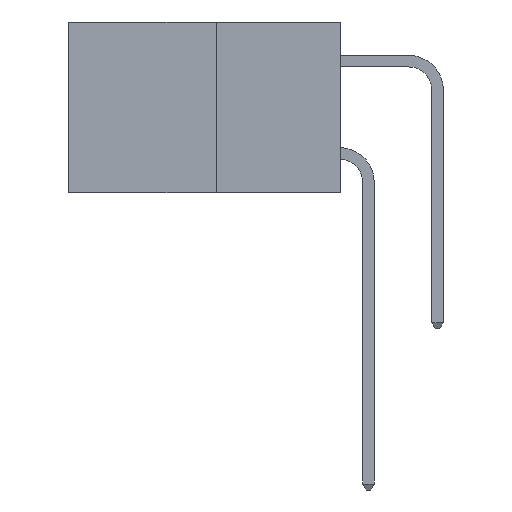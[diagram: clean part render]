
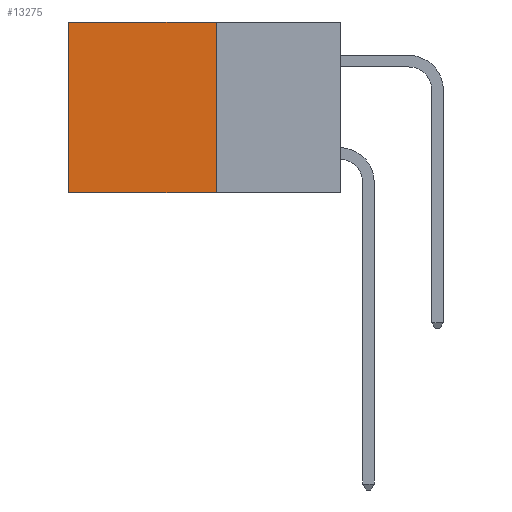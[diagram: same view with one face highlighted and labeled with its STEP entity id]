
A CAD part, left-side view. The second image highlights one B-rep face of the part: STEP entity #13275.
In plain terms, the highlighted planar face has unit normal (-1, 0, 0).
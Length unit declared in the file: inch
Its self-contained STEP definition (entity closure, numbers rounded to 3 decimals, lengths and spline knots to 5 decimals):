
#1402 = DIRECTION ( 'NONE',  ( 0., 0., -1. ) ) ;
#1432 = ORIENTED_EDGE ( 'NONE', *, *, #3267, .T. ) ;
#1830 = VERTEX_POINT ( 'NONE', #9430 ) ;
#2218 = CARTESIAN_POINT ( 'NONE',  ( 0.277, 0.59, -0.37 ) ) ;
#2800 = VERTEX_POINT ( 'NONE', #19745 ) ;
#2997 = VECTOR ( 'NONE', #15778, 39.37008 ) ;
#3267 = EDGE_CURVE ( 'NONE', #7674, #1830, #17263, .T. ) ;
#3533 = PLANE ( 'NONE',  #20308 ) ;
#3918 = FACE_OUTER_BOUND ( 'NONE', #11675, .T. ) ;
#4241 = VERTEX_POINT ( 'NONE', #22824 ) ;
#5569 = CARTESIAN_POINT ( 'NONE',  ( 0.277, 0.27, -0.37 ) ) ;
#5927 = CARTESIAN_POINT ( 'NONE',  ( 0.277, 0.27, 0. ) ) ;
#6633 = DIRECTION ( 'NONE',  ( 0., 1., 0. ) ) ;
#7389 = EDGE_CURVE ( 'NONE', #1830, #4241, #8307, .T. ) ;
#7457 = ORIENTED_EDGE ( 'NONE', *, *, #21465, .F. ) ;
#7630 = DIRECTION ( 'NONE',  ( 1., 0., 0. ) ) ;
#7674 = VERTEX_POINT ( 'NONE', #5927 ) ;
#8307 = LINE ( 'NONE', #2218, #18185 ) ;
#8946 = VECTOR ( 'NONE', #23646, 39.37008 ) ;
#9430 = CARTESIAN_POINT ( 'NONE',  ( 0.277, 0.59, 0. ) ) ;
#11675 = EDGE_LOOP ( 'NONE', ( #17340, #7457, #15820, #1432 ) ) ;
#12660 = VECTOR ( 'NONE', #6633, 39.37008 ) ;
#13275 = ADVANCED_FACE ( 'NONE', ( #3918 ), #3533, .F. ) ;
#13832 = CARTESIAN_POINT ( 'NONE',  ( 0.277, 0.27, -0.37 ) ) ;
#14811 = LINE ( 'NONE', #21645, #8946 ) ;
#15778 = DIRECTION ( 'NONE',  ( 0., 0., -1. ) ) ;
#15820 = ORIENTED_EDGE ( 'NONE', *, *, #20203, .F. ) ;
#17263 = LINE ( 'NONE', #17877, #12660 ) ;
#17340 = ORIENTED_EDGE ( 'NONE', *, *, #7389, .T. ) ;
#17877 = CARTESIAN_POINT ( 'NONE',  ( 0.277, 0.27, 0. ) ) ;
#18185 = VECTOR ( 'NONE', #1402, 39.37008 ) ;
#18250 = LINE ( 'NONE', #13832, #2997 ) ;
#19745 = CARTESIAN_POINT ( 'NONE',  ( 0.277, 0.27, -0.37 ) ) ;
#20203 = EDGE_CURVE ( 'NONE', #7674, #2800, #18250, .T. ) ;
#20308 = AXIS2_PLACEMENT_3D ( 'NONE', #5569, #7630, #21431 ) ;
#21431 = DIRECTION ( 'NONE',  ( 0., 0., -1. ) ) ;
#21465 = EDGE_CURVE ( 'NONE', #2800, #4241, #14811, .T. ) ;
#21645 = CARTESIAN_POINT ( 'NONE',  ( 0.277, 0.27, -0.37 ) ) ;
#22824 = CARTESIAN_POINT ( 'NONE',  ( 0.277, 0.59, -0.37 ) ) ;
#23646 = DIRECTION ( 'NONE',  ( 0., 1., 0. ) ) ;
